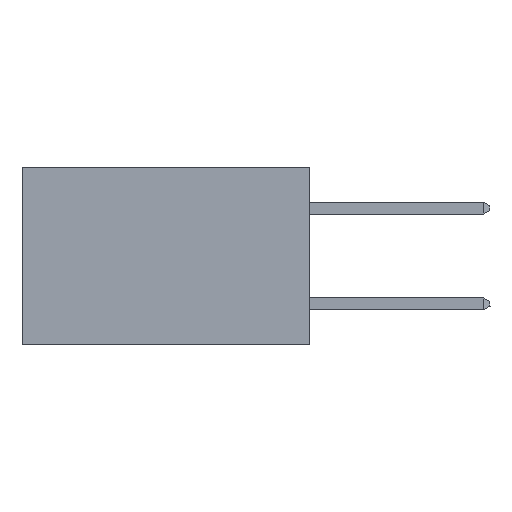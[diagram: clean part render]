
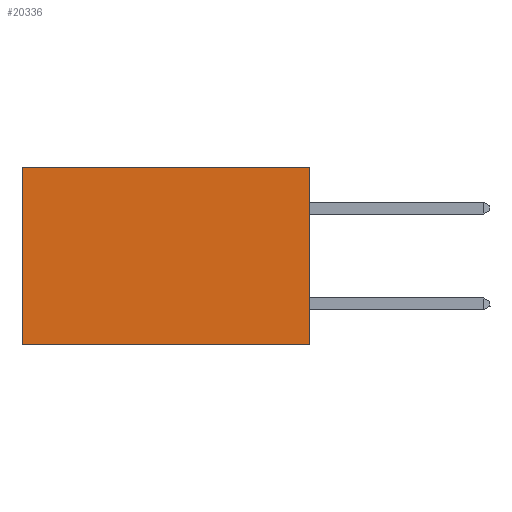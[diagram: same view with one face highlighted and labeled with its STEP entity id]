
A CAD part, left-side view. The second image highlights one B-rep face of the part: STEP entity #20336.
In plain terms, the highlighted planar face has unit normal (-1, 0, 0).
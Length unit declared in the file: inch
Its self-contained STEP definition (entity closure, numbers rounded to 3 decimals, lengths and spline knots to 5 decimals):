
#181 = VERTEX_POINT ( 'NONE', #11253 ) ;
#3497 = AXIS2_PLACEMENT_3D ( 'NONE', #28908, #29259, #34470 ) ;
#4087 = CARTESIAN_POINT ( 'NONE',  ( 0.2875, 0.6, 0. ) ) ;
#4452 = LINE ( 'NONE', #27735, #14684 ) ;
#5099 = CARTESIAN_POINT ( 'NONE',  ( 0.2875, 0.6, 0. ) ) ;
#6130 = DIRECTION ( 'NONE',  ( 0., 0., -1. ) ) ;
#7104 = VERTEX_POINT ( 'NONE', #22583 ) ;
#8667 = DIRECTION ( 'NONE',  ( 0., 1., 0. ) ) ;
#9643 = LINE ( 'NONE', #14478, #17325 ) ;
#10186 = PLANE ( 'NONE',  #3497 ) ;
#10487 = CARTESIAN_POINT ( 'NONE',  ( 0.2875, 0., 0. ) ) ;
#11253 = CARTESIAN_POINT ( 'NONE',  ( 0.2875, 0.6, -0.37 ) ) ;
#12231 = VECTOR ( 'NONE', #29433, 39.37008 ) ;
#13297 = CARTESIAN_POINT ( 'NONE',  ( 0.2875, 0., -0.37 ) ) ;
#14478 = CARTESIAN_POINT ( 'NONE',  ( 0.2875, 0., 0. ) ) ;
#14684 = VECTOR ( 'NONE', #8667, 39.37008 ) ;
#15926 = DIRECTION ( 'NONE',  ( 0., 1., 0. ) ) ;
#16586 = ORIENTED_EDGE ( 'NONE', *, *, #16993, .F. ) ;
#16993 = EDGE_CURVE ( 'NONE', #7104, #181, #20263, .T. ) ;
#17325 = VECTOR ( 'NONE', #6130, 39.37008 ) ;
#19002 = VECTOR ( 'NONE', #15926, 39.37008 ) ;
#19426 = ORIENTED_EDGE ( 'NONE', *, *, #34966, .T. ) ;
#20263 = LINE ( 'NONE', #13297, #19002 ) ;
#20336 = ADVANCED_FACE ( 'NONE', ( #29292 ), #10186, .F. ) ;
#22506 = EDGE_LOOP ( 'NONE', ( #19426, #16586, #31152, #30761 ) ) ;
#22583 = CARTESIAN_POINT ( 'NONE',  ( 0.2875, 0., -0.37 ) ) ;
#22666 = VERTEX_POINT ( 'NONE', #4087 ) ;
#23563 = EDGE_CURVE ( 'NONE', #33817, #22666, #4452, .T. ) ;
#26933 = EDGE_CURVE ( 'NONE', #33817, #7104, #9643, .T. ) ;
#27735 = CARTESIAN_POINT ( 'NONE',  ( 0.2875, 0., 0. ) ) ;
#28441 = LINE ( 'NONE', #5099, #12231 ) ;
#28908 = CARTESIAN_POINT ( 'NONE',  ( 0.2875, 0., 0. ) ) ;
#29259 = DIRECTION ( 'NONE',  ( 1., 0., 0. ) ) ;
#29292 = FACE_OUTER_BOUND ( 'NONE', #22506, .T. ) ;
#29433 = DIRECTION ( 'NONE',  ( 0., 0., -1. ) ) ;
#30761 = ORIENTED_EDGE ( 'NONE', *, *, #23563, .T. ) ;
#31152 = ORIENTED_EDGE ( 'NONE', *, *, #26933, .F. ) ;
#33817 = VERTEX_POINT ( 'NONE', #10487 ) ;
#34470 = DIRECTION ( 'NONE',  ( 0., 0., -1. ) ) ;
#34966 = EDGE_CURVE ( 'NONE', #22666, #181, #28441, .T. ) ;
